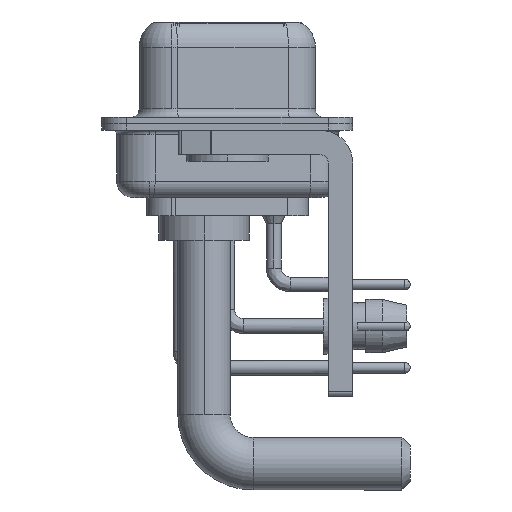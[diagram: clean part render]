
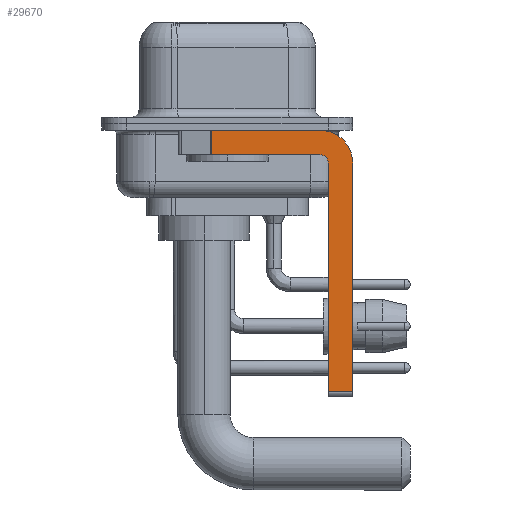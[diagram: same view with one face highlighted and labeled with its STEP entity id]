
A CAD part, left-side view. The second image highlights one B-rep face of the part: STEP entity #29670.
In plain terms, the highlighted planar face has unit normal (-1, 0, 0).
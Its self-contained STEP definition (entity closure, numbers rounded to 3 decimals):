
#18 = VECTOR ( 'NONE', #8687, 1000. ) ;
#201 = CARTESIAN_POINT ( 'NONE',  ( -2.9, 3., -0.4 ) ) ;
#456 = CARTESIAN_POINT ( 'NONE',  ( -2.9, 0.978, -1.9 ) ) ;
#926 = EDGE_CURVE ( 'NONE', #22036, #27674, #21576, .T. ) ;
#2012 = AXIS2_PLACEMENT_3D ( 'NONE', #8614, #30696, #20110 ) ;
#2794 = LINE ( 'NONE', #32650, #28523 ) ;
#3795 = VERTEX_POINT ( 'NONE', #26910 ) ;
#5273 = ORIENTED_EDGE ( 'NONE', *, *, #26303, .F. ) ;
#6158 = EDGE_LOOP ( 'NONE', ( #24494, #15777, #20498, #29514, #19246, #33291, #33806, #5273 ) ) ;
#6180 = CARTESIAN_POINT ( 'NONE',  ( -2.9, -7.65, -2.4 ) ) ;
#6628 = CARTESIAN_POINT ( 'NONE',  ( -2.9, -6.15, -16.35 ) ) ;
#8082 = EDGE_CURVE ( 'NONE', #29621, #3795, #12145, .T. ) ;
#8510 = VERTEX_POINT ( 'NONE', #6628 ) ;
#8614 = CARTESIAN_POINT ( 'NONE',  ( -2.9, -5.65, -2.4 ) ) ;
#8687 = DIRECTION ( 'NONE',  ( 0., -1., 0. ) ) ;
#8820 = DIRECTION ( 'NONE',  ( 0., 0., 1. ) ) ;
#8954 = VERTEX_POINT ( 'NONE', #11717 ) ;
#10053 = VERTEX_POINT ( 'NONE', #30527 ) ;
#11150 = VECTOR ( 'NONE', #26708, 1000. ) ;
#11300 = LINE ( 'NONE', #33018, #28042 ) ;
#11583 = AXIS2_PLACEMENT_3D ( 'NONE', #30562, #24400, #32509 ) ;
#11680 = EDGE_CURVE ( 'NONE', #8510, #27674, #20377, .T. ) ;
#11717 = CARTESIAN_POINT ( 'NONE',  ( -2.9, -5.65, -0.4 ) ) ;
#12145 = CIRCLE ( 'NONE', #11583, 0.5 ) ;
#13599 = DIRECTION ( 'NONE',  ( 0., 1., 0. ) ) ;
#13666 = LINE ( 'NONE', #201, #18 ) ;
#15777 = ORIENTED_EDGE ( 'NONE', *, *, #29979, .T. ) ;
#16214 = LINE ( 'NONE', #456, #18216 ) ;
#17003 = EDGE_CURVE ( 'NONE', #8510, #29621, #11300, .T. ) ;
#18216 = VECTOR ( 'NONE', #19561, 1000. ) ;
#18285 = VECTOR ( 'NONE', #18579, 1000. ) ;
#18579 = DIRECTION ( 'NONE',  ( 0., 0., -1. ) ) ;
#19246 = ORIENTED_EDGE ( 'NONE', *, *, #17003, .F. ) ;
#19561 = DIRECTION ( 'NONE',  ( 0., 0., -1. ) ) ;
#20110 = DIRECTION ( 'NONE',  ( 0., 0., -1. ) ) ;
#20140 = EDGE_CURVE ( 'NONE', #10053, #8954, #13666, .T. ) ;
#20377 = LINE ( 'NONE', #33941, #11150 ) ;
#20481 = DIRECTION ( 'NONE',  ( 1., 0., 0. ) ) ;
#20498 = ORIENTED_EDGE ( 'NONE', *, *, #26274, .F. ) ;
#21077 = CARTESIAN_POINT ( 'NONE',  ( -2.9, -7.65, -16.35 ) ) ;
#21576 = LINE ( 'NONE', #29342, #18285 ) ;
#22036 = VERTEX_POINT ( 'NONE', #6180 ) ;
#23115 = PLANE ( 'NONE',  #24956 ) ;
#24400 = DIRECTION ( 'NONE',  ( -1., 0., 0. ) ) ;
#24494 = ORIENTED_EDGE ( 'NONE', *, *, #20140, .F. ) ;
#24716 = CARTESIAN_POINT ( 'NONE',  ( -2.9, -6.15, -2.4 ) ) ;
#24956 = AXIS2_PLACEMENT_3D ( 'NONE', #33862, #20481, #31229 ) ;
#26274 = EDGE_CURVE ( 'NONE', #3795, #31347, #2794, .T. ) ;
#26303 = EDGE_CURVE ( 'NONE', #8954, #22036, #31923, .T. ) ;
#26708 = DIRECTION ( 'NONE',  ( 0., -1., 0. ) ) ;
#26910 = CARTESIAN_POINT ( 'NONE',  ( -2.9, -5.65, -1.9 ) ) ;
#27674 = VERTEX_POINT ( 'NONE', #21077 ) ;
#28042 = VECTOR ( 'NONE', #8820, 1000. ) ;
#28523 = VECTOR ( 'NONE', #13599, 1000. ) ;
#28838 = CARTESIAN_POINT ( 'NONE',  ( -2.9, 0.978, -1.9 ) ) ;
#29342 = CARTESIAN_POINT ( 'NONE',  ( -2.9, -7.65, -2.4 ) ) ;
#29514 = ORIENTED_EDGE ( 'NONE', *, *, #8082, .F. ) ;
#29621 = VERTEX_POINT ( 'NONE', #24716 ) ;
#29670 = ADVANCED_FACE ( 'NONE', ( #33338 ), #23115, .F. ) ;
#29979 = EDGE_CURVE ( 'NONE', #10053, #31347, #16214, .T. ) ;
#30527 = CARTESIAN_POINT ( 'NONE',  ( -2.9, 0.978, -0.4 ) ) ;
#30562 = CARTESIAN_POINT ( 'NONE',  ( -2.9, -5.65, -2.4 ) ) ;
#30696 = DIRECTION ( 'NONE',  ( 1., 0., 0. ) ) ;
#31229 = DIRECTION ( 'NONE',  ( 0., 0., -1. ) ) ;
#31347 = VERTEX_POINT ( 'NONE', #28838 ) ;
#31923 = CIRCLE ( 'NONE', #2012, 2. ) ;
#32509 = DIRECTION ( 'NONE',  ( 0., 0., 1. ) ) ;
#32650 = CARTESIAN_POINT ( 'NONE',  ( -2.9, -5.65, -1.9 ) ) ;
#33018 = CARTESIAN_POINT ( 'NONE',  ( -2.9, -6.15, -16.6 ) ) ;
#33291 = ORIENTED_EDGE ( 'NONE', *, *, #11680, .T. ) ;
#33338 = FACE_OUTER_BOUND ( 'NONE', #6158, .T. ) ;
#33806 = ORIENTED_EDGE ( 'NONE', *, *, #926, .F. ) ;
#33862 = CARTESIAN_POINT ( 'NONE',  ( -2.9, -5.65, -2.4 ) ) ;
#33941 = CARTESIAN_POINT ( 'NONE',  ( -2.9, -5.65, -16.35 ) ) ;
